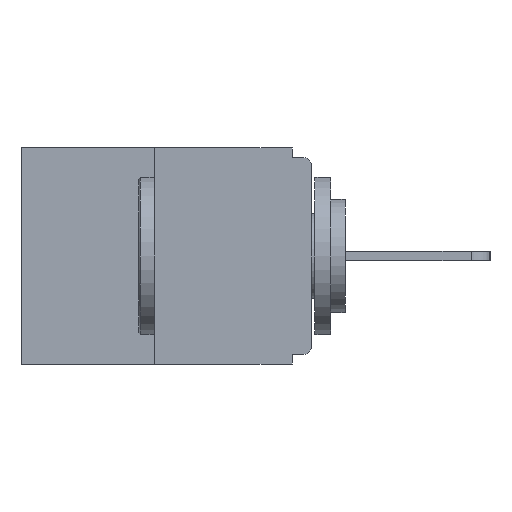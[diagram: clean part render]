
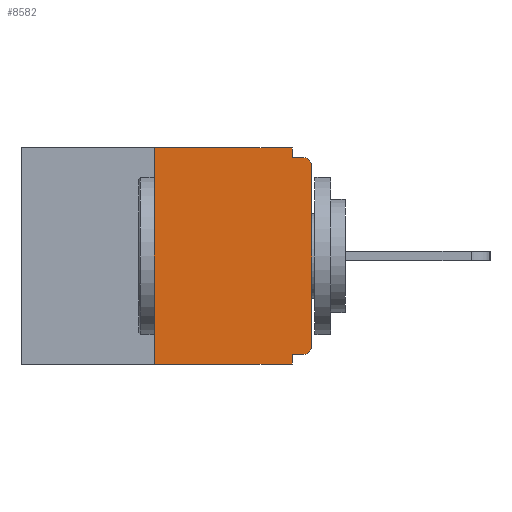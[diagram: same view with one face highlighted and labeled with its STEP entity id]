
A CAD part, left-side view. The second image highlights one B-rep face of the part: STEP entity #8582.
In plain terms, the highlighted planar face has unit normal (-1, 0, 0).
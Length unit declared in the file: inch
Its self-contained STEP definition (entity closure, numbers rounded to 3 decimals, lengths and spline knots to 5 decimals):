
#52 = CARTESIAN_POINT ( 'NONE',  ( 0., 0.031, -0.328 ) ) ;
#905 = EDGE_CURVE ( 'NONE', #13645, #17625, #2300, .T. ) ;
#915 = DIRECTION ( 'NONE',  ( -1., 0., 0. ) ) ;
#1047 = CARTESIAN_POINT ( 'NONE',  ( 0., 0.031, 0. ) ) ;
#1128 = EDGE_CURVE ( 'NONE', #5264, #17102, #12175, .T. ) ;
#1283 = VECTOR ( 'NONE', #17863, 39.37008 ) ;
#1831 = VERTEX_POINT ( 'NONE', #4764 ) ;
#2167 = CARTESIAN_POINT ( 'NONE',  ( 0., 0.031, -0.343 ) ) ;
#2300 = LINE ( 'NONE', #19413, #7990 ) ;
#2568 = CIRCLE ( 'NONE', #12314, 0.015 ) ;
#2574 = CARTESIAN_POINT ( 'NONE',  ( 0., 0.015, -0.015 ) ) ;
#3296 = DIRECTION ( 'NONE',  ( 0., -1., 0. ) ) ;
#3807 = FACE_OUTER_BOUND ( 'NONE', #9005, .T. ) ;
#4395 = ORIENTED_EDGE ( 'NONE', *, *, #1128, .T. ) ;
#4764 = CARTESIAN_POINT ( 'NONE',  ( 0., 0., -0.03 ) ) ;
#5004 = VERTEX_POINT ( 'NONE', #2574 ) ;
#5005 = CARTESIAN_POINT ( 'NONE',  ( 0., 0.46, -0.343 ) ) ;
#5231 = ORIENTED_EDGE ( 'NONE', *, *, #7964, .F. ) ;
#5256 = VECTOR ( 'NONE', #13461, 39.37008 ) ;
#5264 = VERTEX_POINT ( 'NONE', #8607 ) ;
#5601 = CARTESIAN_POINT ( 'NONE',  ( 0., 0., -0.328 ) ) ;
#6149 = DIRECTION ( 'NONE',  ( 0., 0., -1. ) ) ;
#6464 = LINE ( 'NONE', #11283, #12656 ) ;
#7044 = DIRECTION ( 'NONE',  ( 0., 0., -1. ) ) ;
#7047 = EDGE_CURVE ( 'NONE', #10382, #18371, #12368, .T. ) ;
#7322 = VERTEX_POINT ( 'NONE', #7569 ) ;
#7479 = DIRECTION ( 'NONE',  ( -1., 0., 0. ) ) ;
#7569 = CARTESIAN_POINT ( 'NONE',  ( 0., 0.25, 0. ) ) ;
#7964 = EDGE_CURVE ( 'NONE', #19927, #17102, #10656, .T. ) ;
#7990 = VECTOR ( 'NONE', #9533, 39.37008 ) ;
#8159 = DIRECTION ( 'NONE',  ( 0., 0., 1. ) ) ;
#8213 = ORIENTED_EDGE ( 'NONE', *, *, #8818, .F. ) ;
#8559 = CARTESIAN_POINT ( 'NONE',  ( 0., 0., -0.313 ) ) ;
#8582 = ADVANCED_FACE ( 'NONE', ( #3807 ), #18642, .F. ) ;
#8607 = CARTESIAN_POINT ( 'NONE',  ( 0., 0.25, -0.343 ) ) ;
#8705 = ORIENTED_EDGE ( 'NONE', *, *, #19533, .F. ) ;
#8711 = CARTESIAN_POINT ( 'NONE',  ( 0., 0.015, -0.313 ) ) ;
#8818 = EDGE_CURVE ( 'NONE', #17625, #5004, #13623, .T. ) ;
#8920 = DIRECTION ( 'NONE',  ( 0., 1., 0. ) ) ;
#9005 = EDGE_LOOP ( 'NONE', ( #8705, #13193, #4395, #5231, #20341, #20295, #13016, #9127, #8213, #16637 ) ) ;
#9127 = ORIENTED_EDGE ( 'NONE', *, *, #12323, .T. ) ;
#9224 = VECTOR ( 'NONE', #11309, 39.37008 ) ;
#9291 = EDGE_CURVE ( 'NONE', #18371, #1831, #6464, .T. ) ;
#9533 = DIRECTION ( 'NONE',  ( 0., 0., -1. ) ) ;
#9850 = CARTESIAN_POINT ( 'NONE',  ( 0., 0.031, -0.343 ) ) ;
#9935 = VECTOR ( 'NONE', #3296, 39.37008 ) ;
#9990 = CARTESIAN_POINT ( 'NONE',  ( 0., 0., -0.015 ) ) ;
#10382 = VERTEX_POINT ( 'NONE', #12426 ) ;
#10656 = LINE ( 'NONE', #9850, #1283 ) ;
#11283 = CARTESIAN_POINT ( 'NONE',  ( 0., 0., 0. ) ) ;
#11309 = DIRECTION ( 'NONE',  ( 0., -1., 0. ) ) ;
#12175 = LINE ( 'NONE', #5005, #9224 ) ;
#12314 = AXIS2_PLACEMENT_3D ( 'NONE', #13724, #7479, #12362 ) ;
#12323 = EDGE_CURVE ( 'NONE', #1831, #5004, #2568, .T. ) ;
#12362 = DIRECTION ( 'NONE',  ( 0., 0., -1. ) ) ;
#12368 = CIRCLE ( 'NONE', #18952, 0.015 ) ;
#12426 = CARTESIAN_POINT ( 'NONE',  ( 0., 0.015, -0.328 ) ) ;
#12656 = VECTOR ( 'NONE', #17453, 39.37008 ) ;
#12702 = AXIS2_PLACEMENT_3D ( 'NONE', #14095, #15508, #6149 ) ;
#13016 = ORIENTED_EDGE ( 'NONE', *, *, #9291, .T. ) ;
#13193 = ORIENTED_EDGE ( 'NONE', *, *, #17084, .F. ) ;
#13392 = VECTOR ( 'NONE', #8920, 39.37008 ) ;
#13461 = DIRECTION ( 'NONE',  ( 0., -1., 0. ) ) ;
#13516 = LINE ( 'NONE', #15965, #14298 ) ;
#13623 = LINE ( 'NONE', #9990, #5256 ) ;
#13645 = VERTEX_POINT ( 'NONE', #1047 ) ;
#13724 = CARTESIAN_POINT ( 'NONE',  ( 0., 0.015, -0.03 ) ) ;
#14059 = CARTESIAN_POINT ( 'NONE',  ( 0., 0.031, -0.015 ) ) ;
#14095 = CARTESIAN_POINT ( 'NONE',  ( 0., 0.46, 0. ) ) ;
#14298 = VECTOR ( 'NONE', #8159, 39.37008 ) ;
#15508 = DIRECTION ( 'NONE',  ( 1., 0., 0. ) ) ;
#15965 = CARTESIAN_POINT ( 'NONE',  ( 0., 0.25, 0. ) ) ;
#16637 = ORIENTED_EDGE ( 'NONE', *, *, #905, .F. ) ;
#17084 = EDGE_CURVE ( 'NONE', #5264, #7322, #13516, .T. ) ;
#17102 = VERTEX_POINT ( 'NONE', #2167 ) ;
#17311 = LINE ( 'NONE', #5601, #13392 ) ;
#17453 = DIRECTION ( 'NONE',  ( 0., 0., 1. ) ) ;
#17499 = CARTESIAN_POINT ( 'NONE',  ( 0., 0.46, 0. ) ) ;
#17625 = VERTEX_POINT ( 'NONE', #14059 ) ;
#17863 = DIRECTION ( 'NONE',  ( 0., 0., -1. ) ) ;
#18371 = VERTEX_POINT ( 'NONE', #8559 ) ;
#18642 = PLANE ( 'NONE',  #12702 ) ;
#18946 = EDGE_CURVE ( 'NONE', #10382, #19927, #17311, .T. ) ;
#18952 = AXIS2_PLACEMENT_3D ( 'NONE', #8711, #915, #7044 ) ;
#19413 = CARTESIAN_POINT ( 'NONE',  ( 0., 0.031, 0. ) ) ;
#19533 = EDGE_CURVE ( 'NONE', #7322, #13645, #20214, .T. ) ;
#19927 = VERTEX_POINT ( 'NONE', #52 ) ;
#20214 = LINE ( 'NONE', #17499, #9935 ) ;
#20295 = ORIENTED_EDGE ( 'NONE', *, *, #7047, .T. ) ;
#20341 = ORIENTED_EDGE ( 'NONE', *, *, #18946, .F. ) ;
